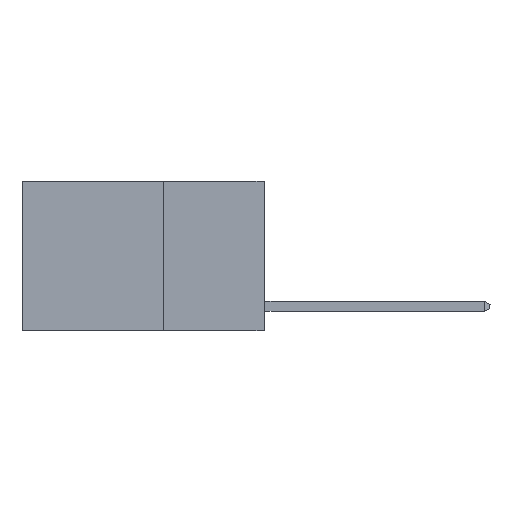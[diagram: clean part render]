
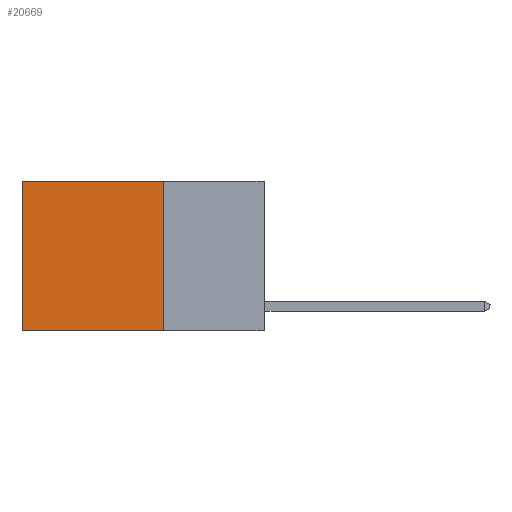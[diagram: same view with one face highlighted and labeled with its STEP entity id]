
A CAD part, left-side view. The second image highlights one B-rep face of the part: STEP entity #20669.
In plain terms, the highlighted planar face has unit normal (-1, 0, 0).
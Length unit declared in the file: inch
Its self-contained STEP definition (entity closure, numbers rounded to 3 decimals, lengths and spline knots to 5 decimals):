
#451 = CARTESIAN_POINT ( 'NONE',  ( 0.2625, 0.25, -0.37 ) ) ;
#1691 = ORIENTED_EDGE ( 'NONE', *, *, #19956, .F. ) ;
#1824 = CARTESIAN_POINT ( 'NONE',  ( 0.2625, 0.25, 0. ) ) ;
#2365 = CARTESIAN_POINT ( 'NONE',  ( 0.2625, 0.25, 0. ) ) ;
#4366 = DIRECTION ( 'NONE',  ( 0., 0., -1. ) ) ;
#5594 = LINE ( 'NONE', #17003, #22966 ) ;
#5799 = EDGE_LOOP ( 'NONE', ( #14924, #9830, #1691, #18143 ) ) ;
#6106 = VECTOR ( 'NONE', #4366, 39.37008 ) ;
#6113 = CARTESIAN_POINT ( 'NONE',  ( 0.2625, 0.6, -0.37 ) ) ;
#6138 = CARTESIAN_POINT ( 'NONE',  ( 0.2625, 0.6, 0. ) ) ;
#8224 = DIRECTION ( 'NONE',  ( 0., 0., -1. ) ) ;
#9532 = VERTEX_POINT ( 'NONE', #11852 ) ;
#9559 = DIRECTION ( 'NONE',  ( 0., 1., 0. ) ) ;
#9830 = ORIENTED_EDGE ( 'NONE', *, *, #22711, .F. ) ;
#10851 = VECTOR ( 'NONE', #9559, 39.37008 ) ;
#11611 = CARTESIAN_POINT ( 'NONE',  ( 0.2625, 0.25, 0. ) ) ;
#11852 = CARTESIAN_POINT ( 'NONE',  ( 0.2625, 0.25, 0. ) ) ;
#14502 = AXIS2_PLACEMENT_3D ( 'NONE', #1824, #23586, #14586 ) ;
#14586 = DIRECTION ( 'NONE',  ( 0., 0., -1. ) ) ;
#14924 = ORIENTED_EDGE ( 'NONE', *, *, #18313, .T. ) ;
#15692 = LINE ( 'NONE', #2365, #10851 ) ;
#16395 = PLANE ( 'NONE',  #14502 ) ;
#17003 = CARTESIAN_POINT ( 'NONE',  ( 0.2625, 0.25, -0.37 ) ) ;
#17392 = VECTOR ( 'NONE', #8224, 39.37008 ) ;
#18143 = ORIENTED_EDGE ( 'NONE', *, *, #20294, .T. ) ;
#18313 = EDGE_CURVE ( 'NONE', #19450, #20043, #22362, .T. ) ;
#19450 = VERTEX_POINT ( 'NONE', #22549 ) ;
#19670 = FACE_OUTER_BOUND ( 'NONE', #5799, .T. ) ;
#19956 = EDGE_CURVE ( 'NONE', #9532, #22185, #21988, .T. ) ;
#20043 = VERTEX_POINT ( 'NONE', #6113 ) ;
#20294 = EDGE_CURVE ( 'NONE', #9532, #19450, #15692, .T. ) ;
#20669 = ADVANCED_FACE ( 'NONE', ( #19670 ), #16395, .F. ) ;
#21988 = LINE ( 'NONE', #11611, #17392 ) ;
#22185 = VERTEX_POINT ( 'NONE', #451 ) ;
#22362 = LINE ( 'NONE', #6138, #6106 ) ;
#22549 = CARTESIAN_POINT ( 'NONE',  ( 0.2625, 0.6, 0. ) ) ;
#22670 = DIRECTION ( 'NONE',  ( 0., 1., 0. ) ) ;
#22711 = EDGE_CURVE ( 'NONE', #22185, #20043, #5594, .T. ) ;
#22966 = VECTOR ( 'NONE', #22670, 39.37008 ) ;
#23586 = DIRECTION ( 'NONE',  ( 1., 0., 0. ) ) ;
